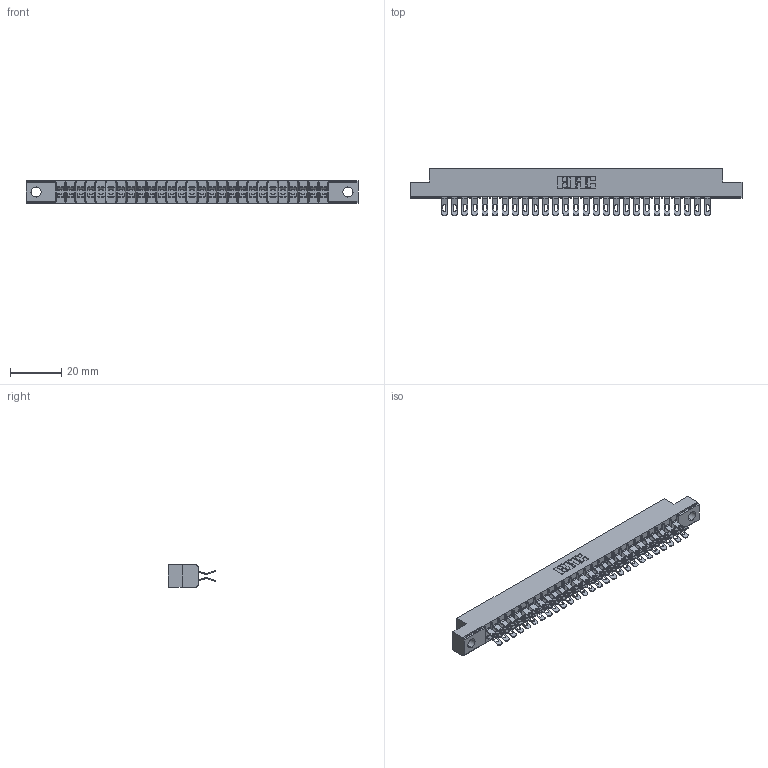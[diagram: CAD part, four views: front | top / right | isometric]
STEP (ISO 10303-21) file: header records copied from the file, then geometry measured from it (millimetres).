
FILE_DESCRIPTION (( 'STEP AP203' ), '1' );
FILE_NAME ('355-054-555-204.STEP', '2019-09-11T17:11:15', ( '' ), ( '' ), 'SwSTEP 2.0', 'SolidWorks 2016', '' );
FILE_SCHEMA (( 'CONFIG_CONTROL_DESIGN' ));
Length unit declared in the file: inch
Products named in the file (3): 305-290-001_555; 305 Part_.156 Dia; 355-054-555-204
Assembly tree (55 placements, depth 2):
  355-054-555-204
    305 Part_.156 Dia
    305-290-001_555  x54
Bounding box: 130 x 18.41 x 8.71 mm (x, y, z)
Volume: 8194.9 mm3; surface area: 16597.1 mm2
Topology: 55 solids, 55 shells, 3694 faces, 11017 edges, 7198 vertices
Faces by surface type: plane 1810, cylinder 1776, sphere 108
Entity records: 32102 total; most frequent: CARTESIAN_POINT 5335, ORIENTED_EDGE 5282, DIRECTION 5159, EDGE_CURVE 2641, VECTOR 2107, LINE 2107, VERTEX_POINT 1686, AXIS2_PLACEMENT_3D 1526
